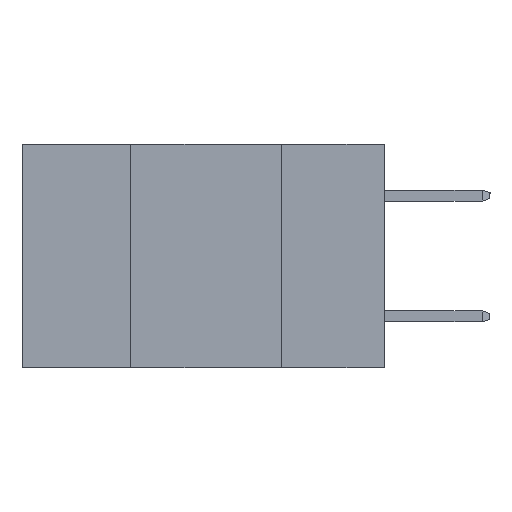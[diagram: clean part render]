
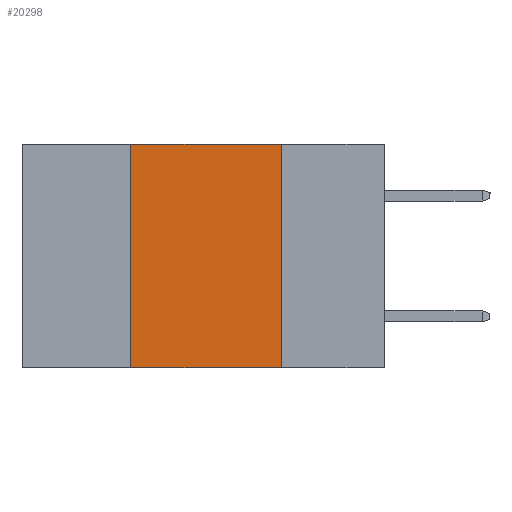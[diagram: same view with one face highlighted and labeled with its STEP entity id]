
A CAD part, left-side view. The second image highlights one B-rep face of the part: STEP entity #20298.
In plain terms, the highlighted planar face has unit normal (-1, 0, 0).
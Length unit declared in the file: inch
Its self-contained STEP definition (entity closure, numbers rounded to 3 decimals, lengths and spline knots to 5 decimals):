
#597 = VERTEX_POINT ( 'NONE', #11198 ) ;
#633 = ORIENTED_EDGE ( 'NONE', *, *, #7661, .F. ) ;
#697 = CARTESIAN_POINT ( 'NONE',  ( 0., 0.42, 0. ) ) ;
#3562 = EDGE_CURVE ( 'NONE', #18968, #8573, #4224, .T. ) ;
#3807 = VERTEX_POINT ( 'NONE', #6628 ) ;
#4224 = LINE ( 'NONE', #10024, #16146 ) ;
#4462 = FACE_OUTER_BOUND ( 'NONE', #20100, .T. ) ;
#4835 = DIRECTION ( 'NONE',  ( 1., 0., 0. ) ) ;
#6462 = CARTESIAN_POINT ( 'NONE',  ( 0., 0.42, -0.37 ) ) ;
#6628 = CARTESIAN_POINT ( 'NONE',  ( 0., 0.42, -0.37 ) ) ;
#7661 = EDGE_CURVE ( 'NONE', #8573, #597, #8149, .T. ) ;
#8149 = LINE ( 'NONE', #17960, #8696 ) ;
#8573 = VERTEX_POINT ( 'NONE', #21638 ) ;
#8696 = VECTOR ( 'NONE', #19343, 39.37008 ) ;
#9168 = ORIENTED_EDGE ( 'NONE', *, *, #3562, .F. ) ;
#10024 = CARTESIAN_POINT ( 'NONE',  ( 0., 0.6, 0. ) ) ;
#10278 = DIRECTION ( 'NONE',  ( 0., -1., 0. ) ) ;
#10582 = AXIS2_PLACEMENT_3D ( 'NONE', #21585, #4835, #16062 ) ;
#10643 = PLANE ( 'NONE',  #10582 ) ;
#11198 = CARTESIAN_POINT ( 'NONE',  ( 0., 0.17, -0.37 ) ) ;
#14560 = ORIENTED_EDGE ( 'NONE', *, *, #23225, .F. ) ;
#16062 = DIRECTION ( 'NONE',  ( 0., 0., -1. ) ) ;
#16146 = VECTOR ( 'NONE', #10278, 39.37008 ) ;
#16156 = CARTESIAN_POINT ( 'NONE',  ( 0., 0.6, -0.37 ) ) ;
#17960 = CARTESIAN_POINT ( 'NONE',  ( 0., 0.17, -0.37 ) ) ;
#18038 = LINE ( 'NONE', #16156, #22161 ) ;
#18968 = VERTEX_POINT ( 'NONE', #697 ) ;
#19343 = DIRECTION ( 'NONE',  ( 0., 0., -1. ) ) ;
#19675 = DIRECTION ( 'NONE',  ( 0., 0., 1. ) ) ;
#20100 = EDGE_LOOP ( 'NONE', ( #633, #9168, #14560, #22936 ) ) ;
#20282 = DIRECTION ( 'NONE',  ( 0., -1., 0. ) ) ;
#20298 = ADVANCED_FACE ( 'NONE', ( #4462 ), #10643, .F. ) ;
#20894 = EDGE_CURVE ( 'NONE', #3807, #597, #18038, .T. ) ;
#21585 = CARTESIAN_POINT ( 'NONE',  ( 0., 0.6, 0. ) ) ;
#21638 = CARTESIAN_POINT ( 'NONE',  ( 0., 0.17, 0. ) ) ;
#22161 = VECTOR ( 'NONE', #20282, 39.37008 ) ;
#22936 = ORIENTED_EDGE ( 'NONE', *, *, #20894, .T. ) ;
#23225 = EDGE_CURVE ( 'NONE', #3807, #18968, #23583, .T. ) ;
#23583 = LINE ( 'NONE', #6462, #23861 ) ;
#23861 = VECTOR ( 'NONE', #19675, 39.37008 ) ;
